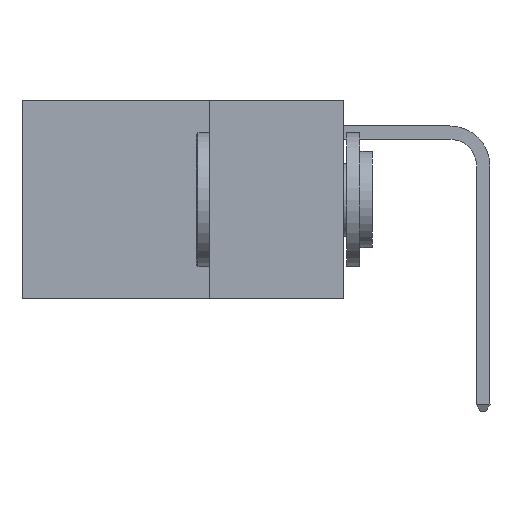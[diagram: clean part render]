
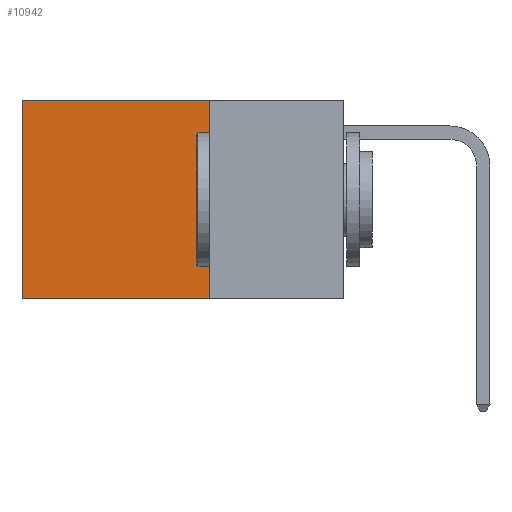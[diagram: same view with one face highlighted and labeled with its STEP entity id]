
A CAD part, left-side view. The second image highlights one B-rep face of the part: STEP entity #10942.
In plain terms, the highlighted planar face has unit normal (-1, 0, 0).
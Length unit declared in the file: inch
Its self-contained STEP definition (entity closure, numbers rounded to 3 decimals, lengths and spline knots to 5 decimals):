
#780 = LINE ( 'NONE', #7202, #6939 ) ;
#848 = VERTEX_POINT ( 'NONE', #10519 ) ;
#2277 = DIRECTION ( 'NONE',  ( 0., 0., -1. ) ) ;
#2483 = DIRECTION ( 'NONE',  ( 0., 0., -1. ) ) ;
#3250 = FACE_OUTER_BOUND ( 'NONE', #11969, .T. ) ;
#3409 = VECTOR ( 'NONE', #2277, 39.37008 ) ;
#3420 = LINE ( 'NONE', #10892, #3409 ) ;
#3660 = ORIENTED_EDGE ( 'NONE', *, *, #8161, .F. ) ;
#4469 = CARTESIAN_POINT ( 'NONE',  ( 0.2625, 0.25, 0. ) ) ;
#4604 = LINE ( 'NONE', #6061, #7892 ) ;
#4850 = DIRECTION ( 'NONE',  ( 0., 1., 0. ) ) ;
#5365 = EDGE_CURVE ( 'NONE', #11861, #7015, #15902, .T. ) ;
#5503 = CARTESIAN_POINT ( 'NONE',  ( 0.2625, 0.6, 0. ) ) ;
#5778 = PLANE ( 'NONE',  #9265 ) ;
#5904 = DIRECTION ( 'NONE',  ( 0., 1., 0. ) ) ;
#6061 = CARTESIAN_POINT ( 'NONE',  ( 0.2625, 0.25, -0.37 ) ) ;
#6939 = VECTOR ( 'NONE', #5904, 39.37008 ) ;
#7015 = VERTEX_POINT ( 'NONE', #8582 ) ;
#7075 = CARTESIAN_POINT ( 'NONE',  ( 0.2625, 0.25, -0.37 ) ) ;
#7202 = CARTESIAN_POINT ( 'NONE',  ( 0.2625, 0.25, 0. ) ) ;
#7322 = ORIENTED_EDGE ( 'NONE', *, *, #13212, .T. ) ;
#7370 = EDGE_CURVE ( 'NONE', #848, #12887, #3420, .T. ) ;
#7892 = VECTOR ( 'NONE', #4850, 39.37008 ) ;
#8161 = EDGE_CURVE ( 'NONE', #12887, #7015, #4604, .T. ) ;
#8283 = ORIENTED_EDGE ( 'NONE', *, *, #7370, .F. ) ;
#8416 = ORIENTED_EDGE ( 'NONE', *, *, #5365, .T. ) ;
#8582 = CARTESIAN_POINT ( 'NONE',  ( 0.2625, 0.6, -0.37 ) ) ;
#9265 = AXIS2_PLACEMENT_3D ( 'NONE', #4469, #9426, #9508 ) ;
#9426 = DIRECTION ( 'NONE',  ( 1., 0., 0. ) ) ;
#9508 = DIRECTION ( 'NONE',  ( 0., 0., -1. ) ) ;
#10269 = CARTESIAN_POINT ( 'NONE',  ( 0.2625, 0.6, 0. ) ) ;
#10519 = CARTESIAN_POINT ( 'NONE',  ( 0.2625, 0.25, 0. ) ) ;
#10892 = CARTESIAN_POINT ( 'NONE',  ( 0.2625, 0.25, 0. ) ) ;
#10942 = ADVANCED_FACE ( 'NONE', ( #3250 ), #5778, .F. ) ;
#11861 = VERTEX_POINT ( 'NONE', #5503 ) ;
#11969 = EDGE_LOOP ( 'NONE', ( #8416, #3660, #8283, #7322 ) ) ;
#12682 = VECTOR ( 'NONE', #2483, 39.37008 ) ;
#12887 = VERTEX_POINT ( 'NONE', #7075 ) ;
#13212 = EDGE_CURVE ( 'NONE', #848, #11861, #780, .T. ) ;
#15902 = LINE ( 'NONE', #10269, #12682 ) ;
